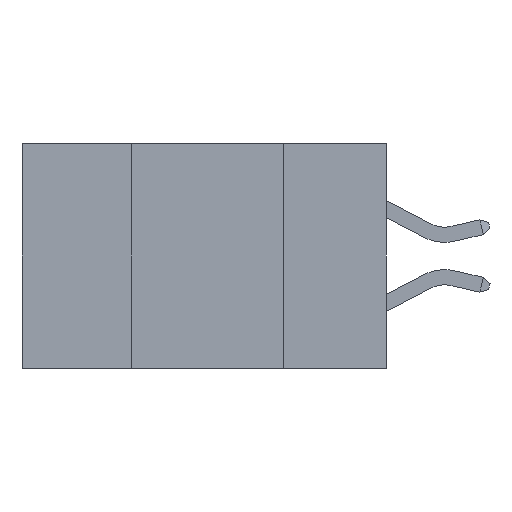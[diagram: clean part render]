
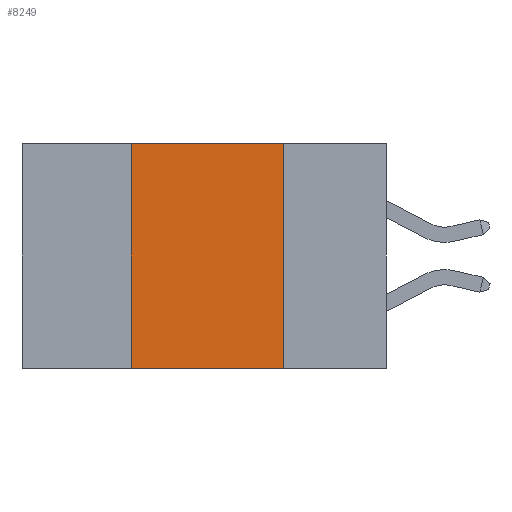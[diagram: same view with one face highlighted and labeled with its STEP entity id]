
A CAD part, left-side view. The second image highlights one B-rep face of the part: STEP entity #8249.
In plain terms, the highlighted planar face has unit normal (-1, 0, 0).
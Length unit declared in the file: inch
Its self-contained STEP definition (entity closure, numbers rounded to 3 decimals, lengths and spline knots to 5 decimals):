
#844 = VERTEX_POINT ( 'NONE', #1205 ) ;
#1205 = CARTESIAN_POINT ( 'NONE',  ( 0., 0.17, -0.37 ) ) ;
#1257 = ORIENTED_EDGE ( 'NONE', *, *, #16236, .T. ) ;
#2175 = VECTOR ( 'NONE', #15021, 39.37008 ) ;
#3072 = CARTESIAN_POINT ( 'NONE',  ( 0., 0.42, -0.37 ) ) ;
#3101 = PLANE ( 'NONE',  #3910 ) ;
#3216 = ORIENTED_EDGE ( 'NONE', *, *, #3577, .F. ) ;
#3359 = DIRECTION ( 'NONE',  ( 0., 0., -1. ) ) ;
#3389 = LINE ( 'NONE', #15334, #3942 ) ;
#3577 = EDGE_CURVE ( 'NONE', #6662, #844, #13867, .T. ) ;
#3910 = AXIS2_PLACEMENT_3D ( 'NONE', #15051, #16705, #6588 ) ;
#3942 = VECTOR ( 'NONE', #5160, 39.37008 ) ;
#5160 = DIRECTION ( 'NONE',  ( 0., -1., 0. ) ) ;
#5484 = CARTESIAN_POINT ( 'NONE',  ( 0., 0.42, 0. ) ) ;
#6588 = DIRECTION ( 'NONE',  ( 0., 0., -1. ) ) ;
#6662 = VERTEX_POINT ( 'NONE', #15688 ) ;
#8249 = ADVANCED_FACE ( 'NONE', ( #19969 ), #3101, .F. ) ;
#8468 = CARTESIAN_POINT ( 'NONE',  ( 0., 0.17, -0.37 ) ) ;
#8536 = CARTESIAN_POINT ( 'NONE',  ( 0., 0.6, 0. ) ) ;
#9357 = VECTOR ( 'NONE', #3359, 39.37008 ) ;
#10246 = DIRECTION ( 'NONE',  ( 0., -1., 0. ) ) ;
#10657 = VECTOR ( 'NONE', #10246, 39.37008 ) ;
#12142 = VERTEX_POINT ( 'NONE', #14198 ) ;
#13867 = LINE ( 'NONE', #8468, #9357 ) ;
#14198 = CARTESIAN_POINT ( 'NONE',  ( 0., 0.42, -0.37 ) ) ;
#15021 = DIRECTION ( 'NONE',  ( 0., 0., 1. ) ) ;
#15051 = CARTESIAN_POINT ( 'NONE',  ( 0., 0.6, 0. ) ) ;
#15240 = LINE ( 'NONE', #3072, #2175 ) ;
#15334 = CARTESIAN_POINT ( 'NONE',  ( 0., 0.6, -0.37 ) ) ;
#15599 = EDGE_LOOP ( 'NONE', ( #3216, #16894, #16745, #1257 ) ) ;
#15672 = EDGE_CURVE ( 'NONE', #19589, #6662, #20071, .T. ) ;
#15688 = CARTESIAN_POINT ( 'NONE',  ( 0., 0.17, 0. ) ) ;
#16236 = EDGE_CURVE ( 'NONE', #12142, #844, #3389, .T. ) ;
#16705 = DIRECTION ( 'NONE',  ( 1., 0., 0. ) ) ;
#16745 = ORIENTED_EDGE ( 'NONE', *, *, #18826, .F. ) ;
#16894 = ORIENTED_EDGE ( 'NONE', *, *, #15672, .F. ) ;
#18826 = EDGE_CURVE ( 'NONE', #12142, #19589, #15240, .T. ) ;
#19589 = VERTEX_POINT ( 'NONE', #5484 ) ;
#19969 = FACE_OUTER_BOUND ( 'NONE', #15599, .T. ) ;
#20071 = LINE ( 'NONE', #8536, #10657 ) ;
